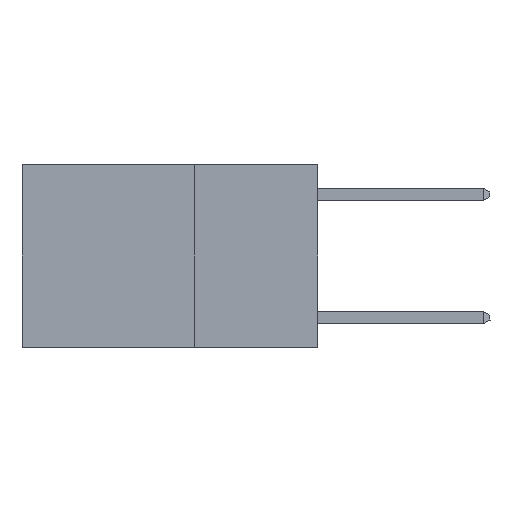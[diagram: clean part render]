
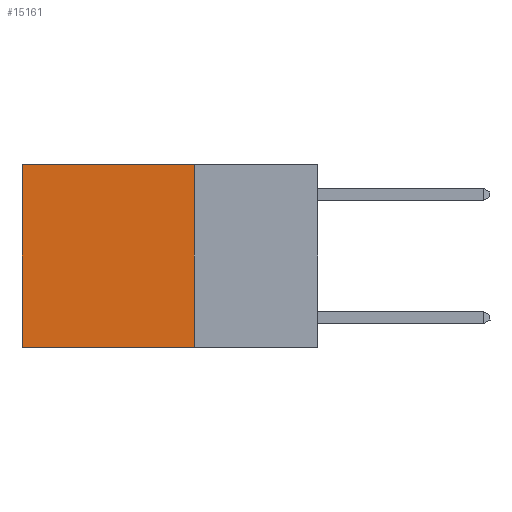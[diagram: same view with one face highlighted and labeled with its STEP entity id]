
A CAD part, left-side view. The second image highlights one B-rep face of the part: STEP entity #15161.
In plain terms, the highlighted planar face has unit normal (-1, 0, 0).
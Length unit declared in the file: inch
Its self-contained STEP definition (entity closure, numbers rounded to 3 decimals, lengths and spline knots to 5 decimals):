
#2101 = VECTOR ( 'NONE', #14560, 39.37008 ) ;
#2302 = CARTESIAN_POINT ( 'NONE',  ( 0.2625, 0.25, 0. ) ) ;
#2647 = EDGE_LOOP ( 'NONE', ( #20624, #3946, #11901, #6018 ) ) ;
#2947 = CARTESIAN_POINT ( 'NONE',  ( 0.2625, 0.6, 0. ) ) ;
#3094 = VECTOR ( 'NONE', #10758, 39.37008 ) ;
#3414 = VERTEX_POINT ( 'NONE', #2302 ) ;
#3508 = DIRECTION ( 'NONE',  ( 0., 1., 0. ) ) ;
#3810 = EDGE_CURVE ( 'NONE', #14304, #14034, #21538, .T. ) ;
#3946 = ORIENTED_EDGE ( 'NONE', *, *, #3810, .F. ) ;
#5978 = CARTESIAN_POINT ( 'NONE',  ( 0.2625, 0.25, 0. ) ) ;
#6018 = ORIENTED_EDGE ( 'NONE', *, *, #7666, .T. ) ;
#7666 = EDGE_CURVE ( 'NONE', #3414, #9782, #8432, .T. ) ;
#7793 = VECTOR ( 'NONE', #23131, 39.37008 ) ;
#7927 = DIRECTION ( 'NONE',  ( 0., 0., -1. ) ) ;
#8432 = LINE ( 'NONE', #9087, #13330 ) ;
#9080 = CARTESIAN_POINT ( 'NONE',  ( 0.2625, 0.25, 0. ) ) ;
#9087 = CARTESIAN_POINT ( 'NONE',  ( 0.2625, 0.25, 0. ) ) ;
#9234 = CARTESIAN_POINT ( 'NONE',  ( 0.2625, 0.25, -0.37 ) ) ;
#9782 = VERTEX_POINT ( 'NONE', #11516 ) ;
#10388 = CARTESIAN_POINT ( 'NONE',  ( 0.2625, 0.6, -0.37 ) ) ;
#10758 = DIRECTION ( 'NONE',  ( 0., 1., 0. ) ) ;
#11516 = CARTESIAN_POINT ( 'NONE',  ( 0.2625, 0.6, 0. ) ) ;
#11901 = ORIENTED_EDGE ( 'NONE', *, *, #14240, .F. ) ;
#13330 = VECTOR ( 'NONE', #3508, 39.37008 ) ;
#14034 = VERTEX_POINT ( 'NONE', #10388 ) ;
#14240 = EDGE_CURVE ( 'NONE', #3414, #14304, #20602, .T. ) ;
#14304 = VERTEX_POINT ( 'NONE', #9234 ) ;
#14560 = DIRECTION ( 'NONE',  ( 0., 0., -1. ) ) ;
#15161 = ADVANCED_FACE ( 'NONE', ( #15975 ), #17122, .F. ) ;
#15975 = FACE_OUTER_BOUND ( 'NONE', #2647, .T. ) ;
#17122 = PLANE ( 'NONE',  #18192 ) ;
#17607 = LINE ( 'NONE', #2947, #7793 ) ;
#18192 = AXIS2_PLACEMENT_3D ( 'NONE', #5978, #18963, #7927 ) ;
#18963 = DIRECTION ( 'NONE',  ( 1., 0., 0. ) ) ;
#20602 = LINE ( 'NONE', #9080, #2101 ) ;
#20624 = ORIENTED_EDGE ( 'NONE', *, *, #22312, .T. ) ;
#21538 = LINE ( 'NONE', #23552, #3094 ) ;
#22312 = EDGE_CURVE ( 'NONE', #9782, #14034, #17607, .T. ) ;
#23131 = DIRECTION ( 'NONE',  ( 0., 0., -1. ) ) ;
#23552 = CARTESIAN_POINT ( 'NONE',  ( 0.2625, 0.25, -0.37 ) ) ;
